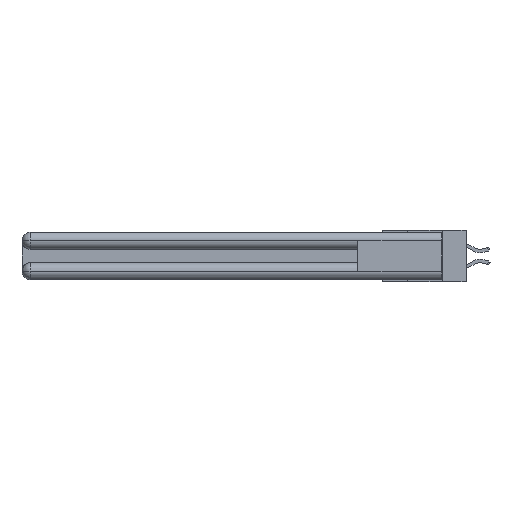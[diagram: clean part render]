
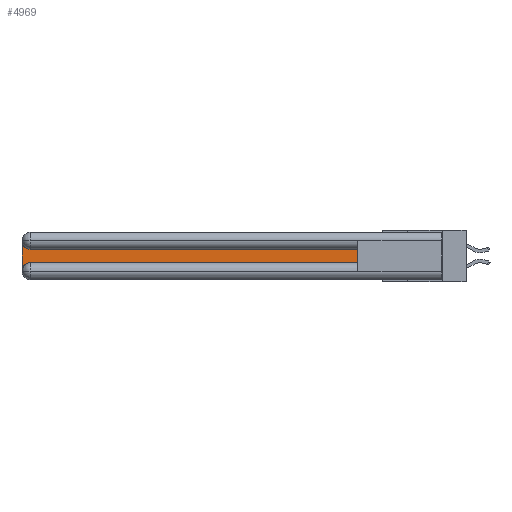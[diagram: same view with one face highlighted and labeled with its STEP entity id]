
A CAD part, left-side view. The second image highlights one B-rep face of the part: STEP entity #4969.
In plain terms, the highlighted planar face has unit normal (-1, 0, 0).
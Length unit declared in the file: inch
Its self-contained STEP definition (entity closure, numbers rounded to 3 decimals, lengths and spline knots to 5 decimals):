
#419 = VERTEX_POINT ( 'NONE', #19923 ) ;
#574 = CARTESIAN_POINT ( 'NONE',  ( 0.075, 0.6, -0.1225 ) ) ;
#739 = AXIS2_PLACEMENT_3D ( 'NONE', #4422, #19836, #15293 ) ;
#859 = EDGE_CURVE ( 'NONE', #2537, #8456, #5242, .T. ) ;
#1015 = CARTESIAN_POINT ( 'NONE',  ( 0.075, 2.94, -0.2775 ) ) ;
#2097 = CARTESIAN_POINT ( 'NONE',  ( 0.075, 0.6, -0.2175 ) ) ;
#2233 = CARTESIAN_POINT ( 'NONE',  ( 0.075, 0.6, -0.2175 ) ) ;
#2537 = VERTEX_POINT ( 'NONE', #11234 ) ;
#2668 = DIRECTION ( 'NONE',  ( 0., 1., 0. ) ) ;
#3486 = LINE ( 'NONE', #26297, #22094 ) ;
#3577 = ORIENTED_EDGE ( 'NONE', *, *, #22290, .T. ) ;
#3868 = DIRECTION ( 'NONE',  ( 1., 0., 0. ) ) ;
#4422 = CARTESIAN_POINT ( 'NONE',  ( 0.075, 2.94, -0.0625 ) ) ;
#4969 = ADVANCED_FACE ( 'NONE', ( #19067 ), #21665, .F. ) ;
#5242 = LINE ( 'NONE', #15702, #27920 ) ;
#5588 = AXIS2_PLACEMENT_3D ( 'NONE', #10672, #3868, #10490 ) ;
#5628 = DIRECTION ( 'NONE',  ( 0., 0., -1. ) ) ;
#8456 = VERTEX_POINT ( 'NONE', #2097 ) ;
#8498 = ORIENTED_EDGE ( 'NONE', *, *, #13232, .T. ) ;
#9542 = EDGE_LOOP ( 'NONE', ( #11475, #8498, #3577, #19802, #23461, #26518 ) ) ;
#10490 = DIRECTION ( 'NONE',  ( 0., 0., -1. ) ) ;
#10672 = CARTESIAN_POINT ( 'NONE',  ( 0.075, 3., -0.1225 ) ) ;
#11106 = EDGE_CURVE ( 'NONE', #13021, #2537, #19387, .T. ) ;
#11234 = CARTESIAN_POINT ( 'NONE',  ( 0.075, 2.94, -0.2175 ) ) ;
#11475 = ORIENTED_EDGE ( 'NONE', *, *, #13577, .T. ) ;
#11617 = CARTESIAN_POINT ( 'NONE',  ( 0.075, 0.6, -0.1225 ) ) ;
#12206 = CARTESIAN_POINT ( 'NONE',  ( 0.075, 3., -0.2775 ) ) ;
#12487 = CARTESIAN_POINT ( 'NONE',  ( 0.075, 2.94, -0.1225 ) ) ;
#13021 = VERTEX_POINT ( 'NONE', #12206 ) ;
#13023 = LINE ( 'NONE', #574, #25419 ) ;
#13232 = EDGE_CURVE ( 'NONE', #23193, #419, #20971, .T. ) ;
#13577 = EDGE_CURVE ( 'NONE', #15746, #23193, #13023, .T. ) ;
#15293 = DIRECTION ( 'NONE',  ( 0., 0., -1. ) ) ;
#15340 = DIRECTION ( 'NONE',  ( 0., 0., -1. ) ) ;
#15702 = CARTESIAN_POINT ( 'NONE',  ( 0.075, 0.6, -0.2175 ) ) ;
#15746 = VERTEX_POINT ( 'NONE', #11617 ) ;
#16578 = DIRECTION ( 'NONE',  ( 1., 0., 0. ) ) ;
#17639 = DIRECTION ( 'NONE',  ( 0., 0., 1. ) ) ;
#19067 = FACE_OUTER_BOUND ( 'NONE', #9542, .T. ) ;
#19387 = CIRCLE ( 'NONE', #23335, 0.06 ) ;
#19646 = LINE ( 'NONE', #2233, #23761 ) ;
#19802 = ORIENTED_EDGE ( 'NONE', *, *, #11106, .T. ) ;
#19836 = DIRECTION ( 'NONE',  ( 1., 0., 0. ) ) ;
#19923 = CARTESIAN_POINT ( 'NONE',  ( 0.075, 3., -0.0625 ) ) ;
#20021 = DIRECTION ( 'NONE',  ( 0., -1., 0. ) ) ;
#20971 = CIRCLE ( 'NONE', #739, 0.06 ) ;
#21665 = PLANE ( 'NONE',  #5588 ) ;
#22094 = VECTOR ( 'NONE', #15340, 39.37008 ) ;
#22290 = EDGE_CURVE ( 'NONE', #419, #13021, #3486, .T. ) ;
#23193 = VERTEX_POINT ( 'NONE', #12487 ) ;
#23335 = AXIS2_PLACEMENT_3D ( 'NONE', #1015, #16578, #5628 ) ;
#23461 = ORIENTED_EDGE ( 'NONE', *, *, #859, .T. ) ;
#23761 = VECTOR ( 'NONE', #17639, 39.37008 ) ;
#23998 = EDGE_CURVE ( 'NONE', #8456, #15746, #19646, .T. ) ;
#25419 = VECTOR ( 'NONE', #2668, 39.37008 ) ;
#26297 = CARTESIAN_POINT ( 'NONE',  ( 0.075, 3., -0.2175 ) ) ;
#26518 = ORIENTED_EDGE ( 'NONE', *, *, #23998, .T. ) ;
#27920 = VECTOR ( 'NONE', #20021, 39.37008 ) ;
